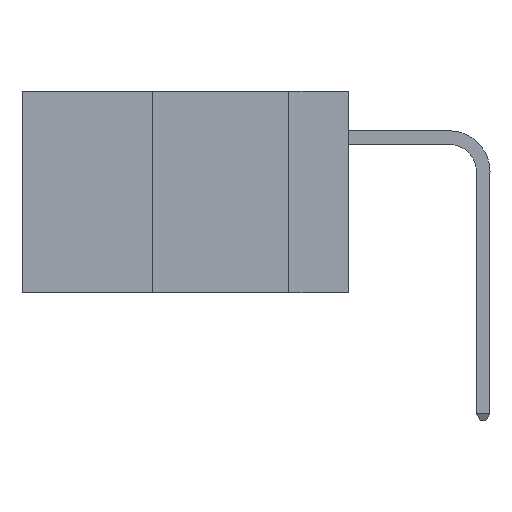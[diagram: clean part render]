
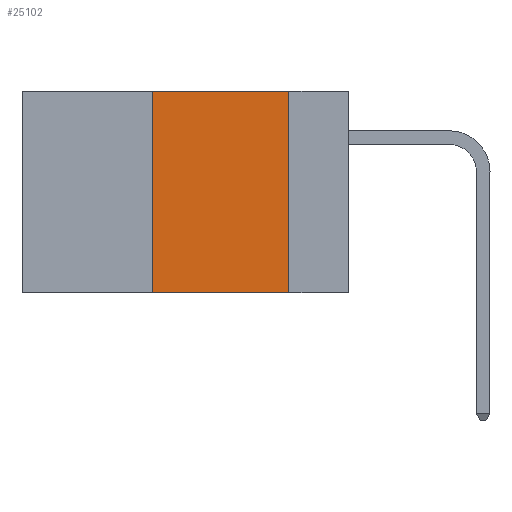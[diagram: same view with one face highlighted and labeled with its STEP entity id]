
A CAD part, left-side view. The second image highlights one B-rep face of the part: STEP entity #25102.
In plain terms, the highlighted planar face has unit normal (-1, 0, 0).
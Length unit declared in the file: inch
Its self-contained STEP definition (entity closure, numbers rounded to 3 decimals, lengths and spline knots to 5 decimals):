
#215 = LINE ( 'NONE', #18578, #29471 ) ;
#869 = DIRECTION ( 'NONE',  ( 0., 0., -1. ) ) ;
#1436 = EDGE_CURVE ( 'NONE', #9879, #16367, #2821, .T. ) ;
#2821 = LINE ( 'NONE', #3614, #13687 ) ;
#2927 = CARTESIAN_POINT ( 'NONE',  ( 0., 0.11, -0.37 ) ) ;
#3614 = CARTESIAN_POINT ( 'NONE',  ( 0., 0.36, 0. ) ) ;
#6213 = VECTOR ( 'NONE', #17278, 39.37008 ) ;
#7639 = EDGE_CURVE ( 'NONE', #17367, #28971, #8796, .T. ) ;
#8796 = LINE ( 'NONE', #12378, #20336 ) ;
#8815 = ORIENTED_EDGE ( 'NONE', *, *, #18078, .T. ) ;
#9130 = CARTESIAN_POINT ( 'NONE',  ( 0., 0.6, 0. ) ) ;
#9310 = DIRECTION ( 'NONE',  ( 0., -1., 0. ) ) ;
#9879 = VERTEX_POINT ( 'NONE', #23097 ) ;
#10587 = DIRECTION ( 'NONE',  ( 0., 0., 1. ) ) ;
#11422 = DIRECTION ( 'NONE',  ( 0., 0., -1. ) ) ;
#12378 = CARTESIAN_POINT ( 'NONE',  ( 0., 0.11, 0. ) ) ;
#13073 = LINE ( 'NONE', #14958, #6213 ) ;
#13687 = VECTOR ( 'NONE', #10587, 39.37008 ) ;
#14958 = CARTESIAN_POINT ( 'NONE',  ( 0., 0.6, -0.37 ) ) ;
#16367 = VERTEX_POINT ( 'NONE', #22448 ) ;
#17278 = DIRECTION ( 'NONE',  ( 0., -1., 0. ) ) ;
#17367 = VERTEX_POINT ( 'NONE', #25820 ) ;
#18078 = EDGE_CURVE ( 'NONE', #9879, #28971, #13073, .T. ) ;
#18578 = CARTESIAN_POINT ( 'NONE',  ( 0., 0.6, 0. ) ) ;
#20336 = VECTOR ( 'NONE', #869, 39.37008 ) ;
#20540 = PLANE ( 'NONE',  #25980 ) ;
#22157 = ORIENTED_EDGE ( 'NONE', *, *, #7639, .F. ) ;
#22448 = CARTESIAN_POINT ( 'NONE',  ( 0., 0.36, 0. ) ) ;
#23097 = CARTESIAN_POINT ( 'NONE',  ( 0., 0.36, -0.37 ) ) ;
#23600 = ORIENTED_EDGE ( 'NONE', *, *, #25153, .F. ) ;
#24831 = FACE_OUTER_BOUND ( 'NONE', #29383, .T. ) ;
#25102 = ADVANCED_FACE ( 'NONE', ( #24831 ), #20540, .F. ) ;
#25153 = EDGE_CURVE ( 'NONE', #16367, #17367, #215, .T. ) ;
#25290 = DIRECTION ( 'NONE',  ( 1., 0., 0. ) ) ;
#25820 = CARTESIAN_POINT ( 'NONE',  ( 0., 0.11, 0. ) ) ;
#25980 = AXIS2_PLACEMENT_3D ( 'NONE', #9130, #25290, #11422 ) ;
#26493 = ORIENTED_EDGE ( 'NONE', *, *, #1436, .F. ) ;
#28971 = VERTEX_POINT ( 'NONE', #2927 ) ;
#29383 = EDGE_LOOP ( 'NONE', ( #22157, #23600, #26493, #8815 ) ) ;
#29471 = VECTOR ( 'NONE', #9310, 39.37008 ) ;
